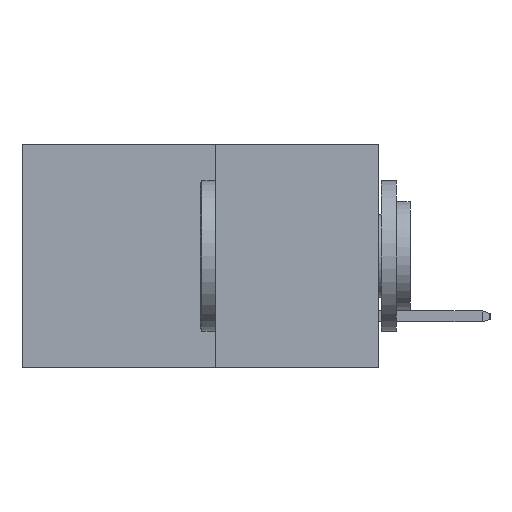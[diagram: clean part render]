
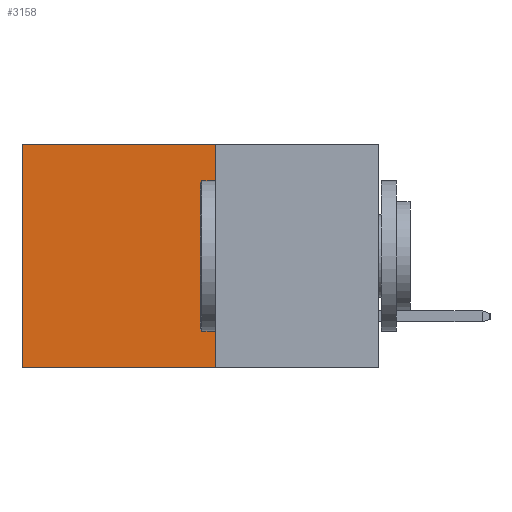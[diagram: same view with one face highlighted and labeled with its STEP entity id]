
A CAD part, left-side view. The second image highlights one B-rep face of the part: STEP entity #3158.
In plain terms, the highlighted planar face has unit normal (-1, 0, 0).
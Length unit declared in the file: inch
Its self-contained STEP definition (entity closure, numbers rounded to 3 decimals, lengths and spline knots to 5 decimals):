
#1200 = CARTESIAN_POINT ( 'NONE',  ( 0.277, 0.27, -0.37 ) ) ;
#1375 = DIRECTION ( 'NONE',  ( 0., 0., -1. ) ) ;
#1718 = VECTOR ( 'NONE', #1375, 39.37008 ) ;
#1747 = VECTOR ( 'NONE', #3524, 39.37008 ) ;
#2081 = LINE ( 'NONE', #1200, #1747 ) ;
#2191 = DIRECTION ( 'NONE',  ( 0., 0., -1. ) ) ;
#2870 = EDGE_CURVE ( 'NONE', #3971, #10227, #2081, .T. ) ;
#3084 = ORIENTED_EDGE ( 'NONE', *, *, #4892, .T. ) ;
#3158 = ADVANCED_FACE ( 'NONE', ( #12617 ), #5767, .F. ) ;
#3524 = DIRECTION ( 'NONE',  ( 0., 1., 0. ) ) ;
#3971 = VERTEX_POINT ( 'NONE', #13597 ) ;
#4892 = EDGE_CURVE ( 'NONE', #12574, #10227, #14084, .T. ) ;
#5008 = LINE ( 'NONE', #5513, #7376 ) ;
#5317 = DIRECTION ( 'NONE',  ( 0., 1., 0. ) ) ;
#5513 = CARTESIAN_POINT ( 'NONE',  ( 0.277, 0.27, 0. ) ) ;
#5522 = CARTESIAN_POINT ( 'NONE',  ( 0.277, 0.59, -0.37 ) ) ;
#5588 = VECTOR ( 'NONE', #7715, 39.37008 ) ;
#5665 = EDGE_CURVE ( 'NONE', #10882, #12574, #5008, .T. ) ;
#5767 = PLANE ( 'NONE',  #13696 ) ;
#6091 = CARTESIAN_POINT ( 'NONE',  ( 0.277, 0.27, -0.37 ) ) ;
#6906 = ORIENTED_EDGE ( 'NONE', *, *, #5665, .T. ) ;
#7376 = VECTOR ( 'NONE', #5317, 39.37008 ) ;
#7715 = DIRECTION ( 'NONE',  ( 0., 0., -1. ) ) ;
#8028 = CARTESIAN_POINT ( 'NONE',  ( 0.277, 0.59, -0.37 ) ) ;
#8195 = CARTESIAN_POINT ( 'NONE',  ( 0.277, 0.27, -0.37 ) ) ;
#9530 = ORIENTED_EDGE ( 'NONE', *, *, #12658, .F. ) ;
#10020 = EDGE_LOOP ( 'NONE', ( #3084, #11980, #9530, #6906 ) ) ;
#10227 = VERTEX_POINT ( 'NONE', #5522 ) ;
#10344 = LINE ( 'NONE', #8195, #1718 ) ;
#10882 = VERTEX_POINT ( 'NONE', #12339 ) ;
#11243 = CARTESIAN_POINT ( 'NONE',  ( 0.277, 0.59, 0. ) ) ;
#11980 = ORIENTED_EDGE ( 'NONE', *, *, #2870, .F. ) ;
#12339 = CARTESIAN_POINT ( 'NONE',  ( 0.277, 0.27, 0. ) ) ;
#12574 = VERTEX_POINT ( 'NONE', #11243 ) ;
#12617 = FACE_OUTER_BOUND ( 'NONE', #10020, .T. ) ;
#12658 = EDGE_CURVE ( 'NONE', #10882, #3971, #10344, .T. ) ;
#13597 = CARTESIAN_POINT ( 'NONE',  ( 0.277, 0.27, -0.37 ) ) ;
#13696 = AXIS2_PLACEMENT_3D ( 'NONE', #6091, #14056, #2191 ) ;
#14056 = DIRECTION ( 'NONE',  ( 1., 0., 0. ) ) ;
#14084 = LINE ( 'NONE', #8028, #5588 ) ;
